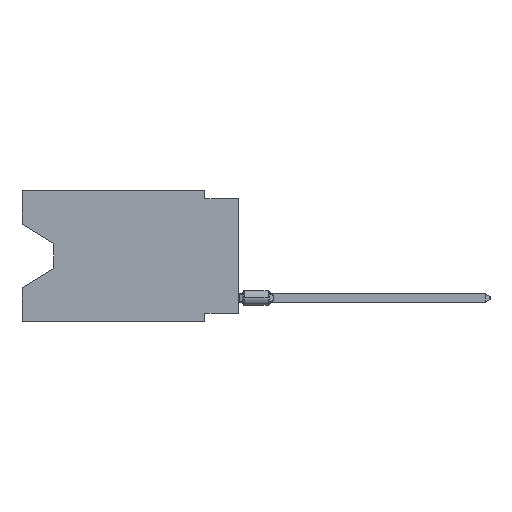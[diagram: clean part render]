
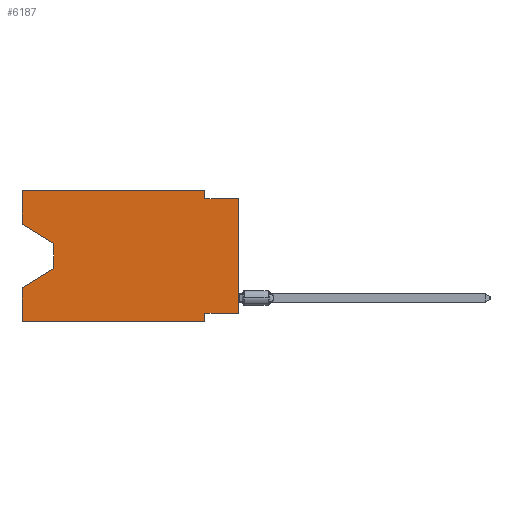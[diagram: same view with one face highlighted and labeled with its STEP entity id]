
A CAD part, left-side view. The second image highlights one B-rep face of the part: STEP entity #6187.
In plain terms, the highlighted planar face has unit normal (-1, 0, 0).
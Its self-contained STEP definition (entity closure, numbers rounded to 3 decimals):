
#351 = CARTESIAN_POINT ( 'NONE',  ( 0., 13.97, -4.013 ) ) ;
#3626 = EDGE_CURVE ( 'NONE', #46504, #12740, #53999, .T. ) ;
#4529 = DIRECTION ( 'NONE',  ( 0., 0., -1. ) ) ;
#5038 = ORIENTED_EDGE ( 'NONE', *, *, #65552, .T. ) ;
#5412 = CARTESIAN_POINT ( 'NONE',  ( 0., 16.383, -7.36 ) ) ;
#5635 = EDGE_CURVE ( 'NONE', #38190, #77013, #24612, .T. ) ;
#6098 = EDGE_CURVE ( 'NONE', #58751, #42562, #63996, .T. ) ;
#6187 = ADVANCED_FACE ( 'NONE', ( #78489 ), #72451, .F. ) ;
#7160 = ORIENTED_EDGE ( 'NONE', *, *, #13795, .F. ) ;
#7817 = CARTESIAN_POINT ( 'NONE',  ( 0., 2.54, 0. ) ) ;
#8577 = CARTESIAN_POINT ( 'NONE',  ( 0., 0., 0. ) ) ;
#9003 = CARTESIAN_POINT ( 'NONE',  ( 0., 2.54, -9.906 ) ) ;
#9405 = CARTESIAN_POINT ( 'NONE',  ( 0., 0., -9.271 ) ) ;
#11540 = DIRECTION ( 'NONE',  ( 0., -1., 0. ) ) ;
#11623 = VECTOR ( 'NONE', #26783, 1000. ) ;
#11898 = ORIENTED_EDGE ( 'NONE', *, *, #6098, .F. ) ;
#12212 = CARTESIAN_POINT ( 'NONE',  ( 0., 16.383, 0. ) ) ;
#12583 = CARTESIAN_POINT ( 'NONE',  ( 0., 13.97, -5.893 ) ) ;
#12740 = VERTEX_POINT ( 'NONE', #53027 ) ;
#13411 = LINE ( 'NONE', #12212, #52288 ) ;
#13795 = EDGE_CURVE ( 'NONE', #32210, #58751, #76498, .T. ) ;
#14700 = DIRECTION ( 'NONE',  ( 0., 0., 1. ) ) ;
#15468 = DIRECTION ( 'NONE',  ( 0., 0., -1. ) ) ;
#16168 = VECTOR ( 'NONE', #37949, 1000. ) ;
#17229 = EDGE_LOOP ( 'NONE', ( #5038, #36686, #78836, #59293, #44646, #11898, #7160, #70877, #54265, #27529, #68280, #66804 ) ) ;
#20455 = VECTOR ( 'NONE', #50841, 1000. ) ;
#20950 = EDGE_CURVE ( 'NONE', #32210, #38326, #38906, .T. ) ;
#22831 = VECTOR ( 'NONE', #51871, 1000. ) ;
#24612 = LINE ( 'NONE', #351, #16168 ) ;
#25283 = VERTEX_POINT ( 'NONE', #5412 ) ;
#26783 = DIRECTION ( 'NONE',  ( 0., 1., 0. ) ) ;
#27529 = ORIENTED_EDGE ( 'NONE', *, *, #61781, .F. ) ;
#28807 = VECTOR ( 'NONE', #11540, 1000. ) ;
#28979 = VECTOR ( 'NONE', #71963, 1000. ) ;
#29671 = CARTESIAN_POINT ( 'NONE',  ( 0., 16.383, 0. ) ) ;
#29677 = CARTESIAN_POINT ( 'NONE',  ( 0., 13.97, -5.893 ) ) ;
#31281 = CARTESIAN_POINT ( 'NONE',  ( 0., 2.54, -9.906 ) ) ;
#32210 = VERTEX_POINT ( 'NONE', #67357 ) ;
#32312 = CARTESIAN_POINT ( 'NONE',  ( 0., 2.54, -9.271 ) ) ;
#32766 = VECTOR ( 'NONE', #14700, 1000. ) ;
#33124 = EDGE_CURVE ( 'NONE', #60944, #42562, #65008, .T. ) ;
#33247 = DIRECTION ( 'NONE',  ( 0., 0., 1. ) ) ;
#33693 = LINE ( 'NONE', #7817, #22831 ) ;
#34217 = EDGE_CURVE ( 'NONE', #77013, #25283, #74032, .T. ) ;
#36686 = ORIENTED_EDGE ( 'NONE', *, *, #5635, .T. ) ;
#37949 = DIRECTION ( 'NONE',  ( 0., 0., -1. ) ) ;
#38190 = VERTEX_POINT ( 'NONE', #74619 ) ;
#38326 = VERTEX_POINT ( 'NONE', #65688 ) ;
#38906 = LINE ( 'NONE', #8577, #45988 ) ;
#38959 = LINE ( 'NONE', #47024, #32766 ) ;
#40757 = CARTESIAN_POINT ( 'NONE',  ( 0., 16.383, -9.906 ) ) ;
#42562 = VERTEX_POINT ( 'NONE', #31281 ) ;
#44646 = ORIENTED_EDGE ( 'NONE', *, *, #33124, .T. ) ;
#45597 = DIRECTION ( 'NONE',  ( 0., -1., 0. ) ) ;
#45988 = VECTOR ( 'NONE', #33247, 1000. ) ;
#46504 = VERTEX_POINT ( 'NONE', #29671 ) ;
#47024 = CARTESIAN_POINT ( 'NONE',  ( 0., 16.383, 0. ) ) ;
#47382 = DIRECTION ( 'NONE',  ( 1., 0., 0. ) ) ;
#49806 = EDGE_CURVE ( 'NONE', #50771, #46504, #13411, .T. ) ;
#50771 = VERTEX_POINT ( 'NONE', #72095 ) ;
#50841 = DIRECTION ( 'NONE',  ( 0., -0.855, -0.519 ) ) ;
#51059 = VECTOR ( 'NONE', #15468, 1000. ) ;
#51871 = DIRECTION ( 'NONE',  ( 0., 0., -1. ) ) ;
#52288 = VECTOR ( 'NONE', #56262, 1000. ) ;
#52526 = VECTOR ( 'NONE', #61506, 1000. ) ;
#53027 = CARTESIAN_POINT ( 'NONE',  ( 0., 2.54, 0. ) ) ;
#53999 = LINE ( 'NONE', #78637, #28807 ) ;
#54265 = ORIENTED_EDGE ( 'NONE', *, *, #70903, .F. ) ;
#56215 = VECTOR ( 'NONE', #45597, 1000. ) ;
#56262 = DIRECTION ( 'NONE',  ( 0., 0., 1. ) ) ;
#57903 = EDGE_CURVE ( 'NONE', #60944, #25283, #38959, .T. ) ;
#58751 = VERTEX_POINT ( 'NONE', #32312 ) ;
#59293 = ORIENTED_EDGE ( 'NONE', *, *, #57903, .F. ) ;
#60944 = VERTEX_POINT ( 'NONE', #40757 ) ;
#61506 = DIRECTION ( 'NONE',  ( 0., 0.855, -0.519 ) ) ;
#61781 = EDGE_CURVE ( 'NONE', #12740, #74548, #33693, .T. ) ;
#62682 = AXIS2_PLACEMENT_3D ( 'NONE', #66789, #47382, #4529 ) ;
#63996 = LINE ( 'NONE', #9003, #51059 ) ;
#65008 = LINE ( 'NONE', #77096, #56215 ) ;
#65552 = EDGE_CURVE ( 'NONE', #50771, #38190, #76692, .T. ) ;
#65688 = CARTESIAN_POINT ( 'NONE',  ( 0., 0., -0.635 ) ) ;
#65901 = CARTESIAN_POINT ( 'NONE',  ( 0., 0., -0.635 ) ) ;
#66789 = CARTESIAN_POINT ( 'NONE',  ( 0., 16.383, 0. ) ) ;
#66804 = ORIENTED_EDGE ( 'NONE', *, *, #49806, .F. ) ;
#67357 = CARTESIAN_POINT ( 'NONE',  ( 0., 0., -9.271 ) ) ;
#68280 = ORIENTED_EDGE ( 'NONE', *, *, #3626, .F. ) ;
#68492 = CARTESIAN_POINT ( 'NONE',  ( 0., 2.54, -0.635 ) ) ;
#69435 = CARTESIAN_POINT ( 'NONE',  ( 0., 16.383, -2.546 ) ) ;
#70877 = ORIENTED_EDGE ( 'NONE', *, *, #20950, .T. ) ;
#70903 = EDGE_CURVE ( 'NONE', #74548, #38326, #78007, .T. ) ;
#71963 = DIRECTION ( 'NONE',  ( 0., -1., 0. ) ) ;
#72095 = CARTESIAN_POINT ( 'NONE',  ( 0., 16.383, -2.546 ) ) ;
#72451 = PLANE ( 'NONE',  #62682 ) ;
#74032 = LINE ( 'NONE', #12583, #52526 ) ;
#74548 = VERTEX_POINT ( 'NONE', #68492 ) ;
#74619 = CARTESIAN_POINT ( 'NONE',  ( 0., 13.97, -4.013 ) ) ;
#76498 = LINE ( 'NONE', #9405, #11623 ) ;
#76692 = LINE ( 'NONE', #69435, #20455 ) ;
#77013 = VERTEX_POINT ( 'NONE', #29677 ) ;
#77096 = CARTESIAN_POINT ( 'NONE',  ( 0., 16.383, -9.906 ) ) ;
#78007 = LINE ( 'NONE', #65901, #28979 ) ;
#78489 = FACE_OUTER_BOUND ( 'NONE', #17229, .T. ) ;
#78637 = CARTESIAN_POINT ( 'NONE',  ( 0., 16.383, 0. ) ) ;
#78836 = ORIENTED_EDGE ( 'NONE', *, *, #34217, .T. ) ;
